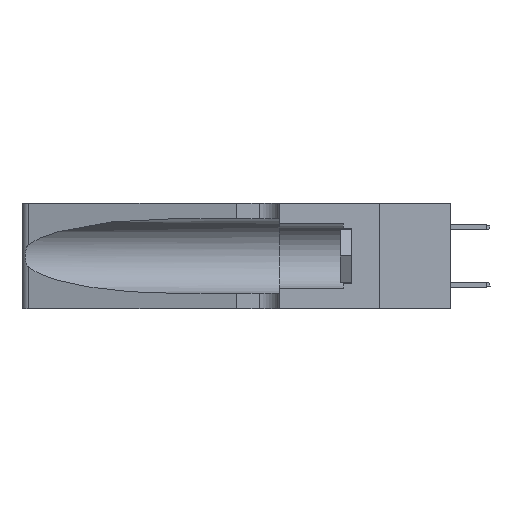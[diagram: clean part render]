
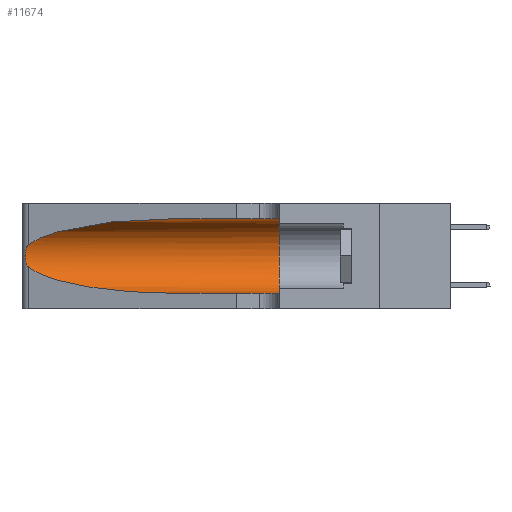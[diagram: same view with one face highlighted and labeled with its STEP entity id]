
A CAD part, left-side view. The second image highlights one B-rep face of the part: STEP entity #11674.
In plain terms, the highlighted cylindrical face has radius 3.308 mm (diameter 6.617 mm), a partial arc.
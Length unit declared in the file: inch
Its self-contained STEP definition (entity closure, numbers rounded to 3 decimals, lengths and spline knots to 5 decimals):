
#89 = CARTESIAN_POINT ( 'NONE',  ( 0.1305, 0.35, 0.05475 ) ) ;
#454 = EDGE_CURVE ( 'NONE', #8089, #5886, #11561, .T. ) ;
#576 = EDGE_CURVE ( 'NONE', #10015, #8089, #10323, .T. ) ;
#812 = AXIS2_PLACEMENT_3D ( 'NONE', #13954, #3483, #2260 ) ;
#968 = ORIENTED_EDGE ( 'NONE', *, *, #7499, .T. ) ;
#1021 = DIRECTION ( 'NONE',  ( 0., 0., -1. ) ) ;
#1263 = CARTESIAN_POINT ( 'NONE',  ( 0.25856, 1.23593, 0.16098 ) ) ;
#1521 = CARTESIAN_POINT ( 'NONE',  ( 0.25555, 1.22994, 0.2215 ) ) ;
#1601 = CARTESIAN_POINT ( 'NONE',  ( 0.25854, 1.2359, 0.20912 ) ) ;
#2187 = ORIENTED_EDGE ( 'NONE', *, *, #13254, .T. ) ;
#2260 = DIRECTION ( 'NONE',  ( 0., 0., 1. ) ) ;
#2266 = EDGE_CURVE ( 'NONE', #16784, #14802, #13675, .T. ) ;
#2326 = CARTESIAN_POINT ( 'NONE',  ( 0.18966, 0.96281, 0.05475 ) ) ;
#3297 = CARTESIAN_POINT ( 'NONE',  ( 0.2373, 1.15595, 0.28018 ) ) ;
#3483 = DIRECTION ( 'NONE',  ( 0., 1., 0. ) ) ;
#4949 = CARTESIAN_POINT ( 'NONE',  ( 0.1305, 1.61858, 0.31525 ) ) ;
#5267 = CARTESIAN_POINT ( 'NONE',  ( 0.25487, 1.22718, 0.14631 ) ) ;
#5611 = CARTESIAN_POINT ( 'NONE',  ( 0.26018, 1.23835, 0.19895 ) ) ;
#5689 = EDGE_CURVE ( 'NONE', #9764, #5886, #16893, .T. ) ;
#5886 = VERTEX_POINT ( 'NONE', #89 ) ;
#6543 = CARTESIAN_POINT ( 'NONE',  ( 0.25487, 1.22718, 0.22369 ) ) ;
#6732 = CARTESIAN_POINT ( 'NONE',  ( 0.25487, 1.22718, 0.14631 ) ) ;
#7434 = CARTESIAN_POINT ( 'NONE',  ( 0.1305, 0.72297, 0.05475 ) ) ;
#7497 = CARTESIAN_POINT ( 'NONE',  ( 0.25487, 1.22718, 0.14631 ) ) ;
#7499 = EDGE_CURVE ( 'NONE', #14802, #9764, #14044, .T. ) ;
#7578 = CARTESIAN_POINT ( 'NONE',  ( 0.1305, 0.72297, 0.05475 ) ) ;
#7760 = CARTESIAN_POINT ( 'NONE',  ( 0.1305, 1.61858, 0.05475 ) ) ;
#7817 = CARTESIAN_POINT ( 'NONE',  ( 0.25787, 1.23484, 0.2124 ) ) ;
#8089 = VERTEX_POINT ( 'NONE', #11393 ) ;
#8278 = AXIS2_PLACEMENT_3D ( 'NONE', #16879, #11358, #1021 ) ;
#8620 = CARTESIAN_POINT ( 'NONE',  ( 0.25487, 1.22718, 0.22369 ) ) ;
#8748 = CARTESIAN_POINT ( 'NONE',  ( 0.25639, 1.23186, 0.15144 ) ) ;
#9019 = FACE_OUTER_BOUND ( 'NONE', #13843, .T. ) ;
#9197 =( BOUNDED_CURVE ( )  B_SPLINE_CURVE ( 3, ( #15329, #12576, #3297, #10143 ),
 .UNSPECIFIED., .F., .T. ) 
 B_SPLINE_CURVE_WITH_KNOTS ( ( 4, 4 ),
 ( 1.5708, 2.84003 ),
 .UNSPECIFIED. ) 
 CURVE ( )  GEOMETRIC_REPRESENTATION_ITEM ( )  RATIONAL_B_SPLINE_CURVE ( ( 1., 0.87, 0.87, 1. ) ) 
 REPRESENTATION_ITEM ( '' )  );
#9764 = VERTEX_POINT ( 'NONE', #7434 ) ;
#10015 = VERTEX_POINT ( 'NONE', #13176 ) ;
#10140 = CARTESIAN_POINT ( 'NONE',  ( 0.2373, 1.15595, 0.08982 ) ) ;
#10143 = CARTESIAN_POINT ( 'NONE',  ( 0.25487, 1.22718, 0.22369 ) ) ;
#10323 = LINE ( 'NONE', #4949, #10724 ) ;
#10724 = VECTOR ( 'NONE', #13255, 39.37008 ) ;
#11358 = DIRECTION ( 'NONE',  ( 0., -1., 0. ) ) ;
#11393 = CARTESIAN_POINT ( 'NONE',  ( 0.1305, 0.35, 0.31525 ) ) ;
#11561 = CIRCLE ( 'NONE', #812, 0.13025 ) ;
#11674 = ADVANCED_FACE ( 'NONE', ( #9019 ), #13075, .F. ) ;
#11778 = CARTESIAN_POINT ( 'NONE',  ( 0.25789, 1.23486, 0.15765 ) ) ;
#11866 = CARTESIAN_POINT ( 'NONE',  ( 0.25639, 1.23184, 0.21858 ) ) ;
#12576 = CARTESIAN_POINT ( 'NONE',  ( 0.18966, 0.96281, 0.31525 ) ) ;
#13061 = CARTESIAN_POINT ( 'NONE',  ( 0.26075, 1.23896, 0.178 ) ) ;
#13075 = CYLINDRICAL_SURFACE ( 'NONE', #8278, 0.13025 ) ;
#13146 = CARTESIAN_POINT ( 'NONE',  ( 0.26075, 1.23896, 0.19203 ) ) ;
#13176 = CARTESIAN_POINT ( 'NONE',  ( 0.1305, 0.72297, 0.31525 ) ) ;
#13254 = EDGE_CURVE ( 'NONE', #10015, #16784, #9197, .T. ) ;
#13255 = DIRECTION ( 'NONE',  ( 0., -1., 0. ) ) ;
#13302 = ORIENTED_EDGE ( 'NONE', *, *, #576, .F. ) ;
#13341 = ORIENTED_EDGE ( 'NONE', *, *, #454, .F. ) ;
#13675 = B_SPLINE_CURVE_WITH_KNOTS ( 'NONE', 3,
 ( #6543, #1521, #11866, #7817, #1601, #5611, #13146, #13061, #15661, #1263, #11778, #8748, #15988, #5267 ),
 .UNSPECIFIED., .F., .F.,
 ( 4, 2, 2, 2, 2, 2, 4 ),
 ( 0., 0.00027, 0.00053, 0.00107, 0.0016, 0.00187, 0.00214 ),
 .UNSPECIFIED. ) ;
#13843 = EDGE_LOOP ( 'NONE', ( #2187, #15776, #968, #15894, #13341, #13302 ) ) ;
#13954 = CARTESIAN_POINT ( 'NONE',  ( 0.1305, 0.35, 0.185 ) ) ;
#14044 =( BOUNDED_CURVE ( )  B_SPLINE_CURVE ( 3, ( #7497, #10140, #2326, #7578 ),
 .UNSPECIFIED., .F., .T. ) 
 B_SPLINE_CURVE_WITH_KNOTS ( ( 4, 4 ),
 ( 3.44316, 4.71239 ),
 .UNSPECIFIED. ) 
 CURVE ( )  GEOMETRIC_REPRESENTATION_ITEM ( )  RATIONAL_B_SPLINE_CURVE ( ( 1., 0.87, 0.87, 1. ) ) 
 REPRESENTATION_ITEM ( '' )  );
#14217 = DIRECTION ( 'NONE',  ( 0., -1., 0. ) ) ;
#14802 = VERTEX_POINT ( 'NONE', #6732 ) ;
#15329 = CARTESIAN_POINT ( 'NONE',  ( 0.1305, 0.72297, 0.31525 ) ) ;
#15661 = CARTESIAN_POINT ( 'NONE',  ( 0.26017, 1.23833, 0.17102 ) ) ;
#15776 = ORIENTED_EDGE ( 'NONE', *, *, #2266, .T. ) ;
#15894 = ORIENTED_EDGE ( 'NONE', *, *, #5689, .T. ) ;
#15988 = CARTESIAN_POINT ( 'NONE',  ( 0.25555, 1.22993, 0.14849 ) ) ;
#16417 = VECTOR ( 'NONE', #14217, 39.37008 ) ;
#16784 = VERTEX_POINT ( 'NONE', #8620 ) ;
#16879 = CARTESIAN_POINT ( 'NONE',  ( 0.1305, 1.61858, 0.185 ) ) ;
#16893 = LINE ( 'NONE', #7760, #16417 ) ;
